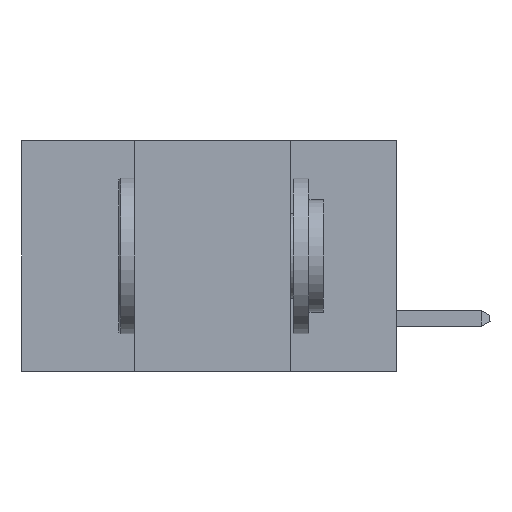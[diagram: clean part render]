
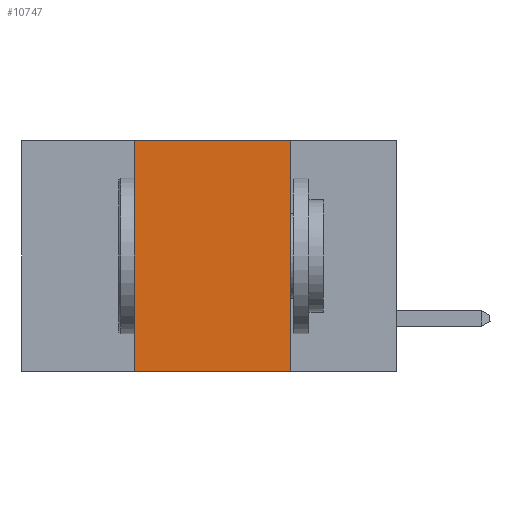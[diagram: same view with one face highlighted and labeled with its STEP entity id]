
A CAD part, left-side view. The second image highlights one B-rep face of the part: STEP entity #10747.
In plain terms, the highlighted planar face has unit normal (-1, 0, 0).
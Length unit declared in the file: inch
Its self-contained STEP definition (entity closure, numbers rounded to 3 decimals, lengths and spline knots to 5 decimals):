
#516 = VECTOR ( 'NONE', #3402, 39.37008 ) ;
#1336 = CARTESIAN_POINT ( 'NONE',  ( 0., 0.17, -0.37 ) ) ;
#1647 = CARTESIAN_POINT ( 'NONE',  ( 0., 0.42, 0. ) ) ;
#1853 = EDGE_CURVE ( 'NONE', #4575, #8251, #2818, .T. ) ;
#2546 = CARTESIAN_POINT ( 'NONE',  ( 0., 0.6, -0.37 ) ) ;
#2659 = VERTEX_POINT ( 'NONE', #1336 ) ;
#2818 = LINE ( 'NONE', #10485, #11045 ) ;
#3395 = ORIENTED_EDGE ( 'NONE', *, *, #1853, .F. ) ;
#3402 = DIRECTION ( 'NONE',  ( 0., -1., 0. ) ) ;
#3624 = FACE_OUTER_BOUND ( 'NONE', #4983, .T. ) ;
#3665 = AXIS2_PLACEMENT_3D ( 'NONE', #4223, #10234, #5120 ) ;
#3675 = LINE ( 'NONE', #2546, #516 ) ;
#4223 = CARTESIAN_POINT ( 'NONE',  ( 0., 0.6, 0. ) ) ;
#4252 = ORIENTED_EDGE ( 'NONE', *, *, #8742, .T. ) ;
#4575 = VERTEX_POINT ( 'NONE', #1647 ) ;
#4983 = EDGE_LOOP ( 'NONE', ( #8303, #3395, #10197, #4252 ) ) ;
#5120 = DIRECTION ( 'NONE',  ( 0., 0., -1. ) ) ;
#5246 = EDGE_CURVE ( 'NONE', #8251, #2659, #8156, .T. ) ;
#6323 = CARTESIAN_POINT ( 'NONE',  ( 0., 0.42, -0.37 ) ) ;
#6544 = LINE ( 'NONE', #10366, #8567 ) ;
#7130 = VERTEX_POINT ( 'NONE', #6323 ) ;
#8156 = LINE ( 'NONE', #8798, #10362 ) ;
#8164 = EDGE_CURVE ( 'NONE', #7130, #4575, #6544, .T. ) ;
#8251 = VERTEX_POINT ( 'NONE', #10481 ) ;
#8303 = ORIENTED_EDGE ( 'NONE', *, *, #5246, .F. ) ;
#8423 = DIRECTION ( 'NONE',  ( 0., -1., 0. ) ) ;
#8567 = VECTOR ( 'NONE', #11152, 39.37008 ) ;
#8583 = PLANE ( 'NONE',  #3665 ) ;
#8742 = EDGE_CURVE ( 'NONE', #7130, #2659, #3675, .T. ) ;
#8798 = CARTESIAN_POINT ( 'NONE',  ( 0., 0.17, 0. ) ) ;
#9591 = DIRECTION ( 'NONE',  ( 0., 0., -1. ) ) ;
#10197 = ORIENTED_EDGE ( 'NONE', *, *, #8164, .F. ) ;
#10234 = DIRECTION ( 'NONE',  ( 1., 0., 0. ) ) ;
#10362 = VECTOR ( 'NONE', #9591, 39.37008 ) ;
#10366 = CARTESIAN_POINT ( 'NONE',  ( 0., 0.42, 0. ) ) ;
#10481 = CARTESIAN_POINT ( 'NONE',  ( 0., 0.17, 0. ) ) ;
#10485 = CARTESIAN_POINT ( 'NONE',  ( 0., 0.6, 0. ) ) ;
#10747 = ADVANCED_FACE ( 'NONE', ( #3624 ), #8583, .F. ) ;
#11045 = VECTOR ( 'NONE', #8423, 39.37008 ) ;
#11152 = DIRECTION ( 'NONE',  ( 0., 0., 1. ) ) ;
